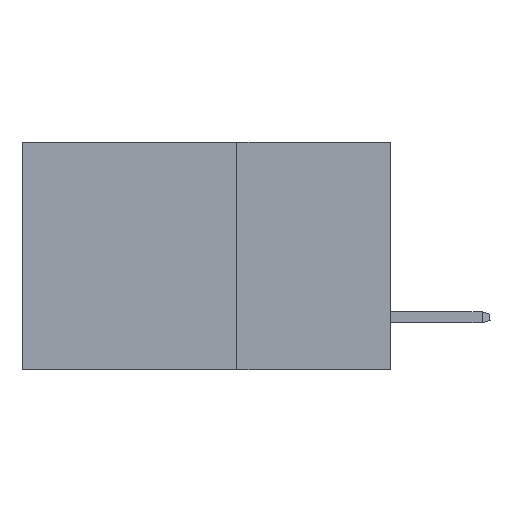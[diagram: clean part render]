
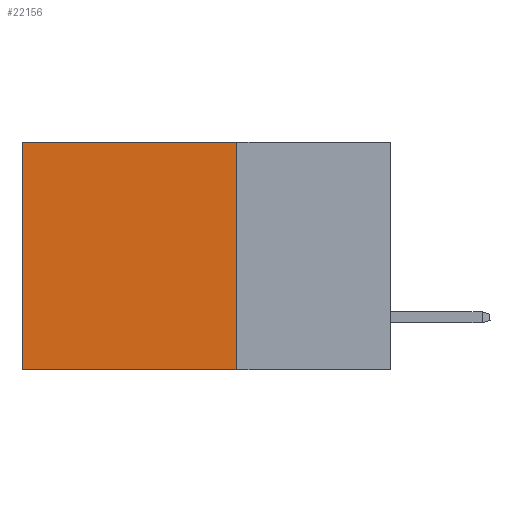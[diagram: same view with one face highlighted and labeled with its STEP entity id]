
A CAD part, left-side view. The second image highlights one B-rep face of the part: STEP entity #22156.
In plain terms, the highlighted planar face has unit normal (-1, 0, 0).
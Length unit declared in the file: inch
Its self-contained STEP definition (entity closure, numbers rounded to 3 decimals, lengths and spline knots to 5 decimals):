
#154 = LINE ( 'NONE', #38061, #28323 ) ;
#233 = CARTESIAN_POINT ( 'NONE',  ( 0.2875, 0.25, 0. ) ) ;
#596 = DIRECTION ( 'NONE',  ( 1., 0., 0. ) ) ;
#2822 = DIRECTION ( 'NONE',  ( 0., 1., 0. ) ) ;
#3446 = AXIS2_PLACEMENT_3D ( 'NONE', #34140, #596, #27820 ) ;
#3474 = ORIENTED_EDGE ( 'NONE', *, *, #25304, .T. ) ;
#4267 = CARTESIAN_POINT ( 'NONE',  ( 0.2875, 0.6, 0. ) ) ;
#4730 = ORIENTED_EDGE ( 'NONE', *, *, #14079, .F. ) ;
#5203 = CARTESIAN_POINT ( 'NONE',  ( 0.2875, 0.6, -0.37 ) ) ;
#5903 = CARTESIAN_POINT ( 'NONE',  ( 0.2875, 0.25, 0. ) ) ;
#7310 = DIRECTION ( 'NONE',  ( 0., 0., -1. ) ) ;
#7563 = LINE ( 'NONE', #25969, #22406 ) ;
#9550 = EDGE_CURVE ( 'NONE', #39349, #24073, #13376, .T. ) ;
#11528 = FACE_OUTER_BOUND ( 'NONE', #12274, .T. ) ;
#12274 = EDGE_LOOP ( 'NONE', ( #20161, #17714, #4730, #3474 ) ) ;
#12705 = CARTESIAN_POINT ( 'NONE',  ( 0.2875, 0.6, 0. ) ) ;
#13376 = LINE ( 'NONE', #4267, #39272 ) ;
#14079 = EDGE_CURVE ( 'NONE', #20731, #23563, #7563, .T. ) ;
#16460 = VECTOR ( 'NONE', #2822, 39.37008 ) ;
#17714 = ORIENTED_EDGE ( 'NONE', *, *, #30950, .F. ) ;
#20161 = ORIENTED_EDGE ( 'NONE', *, *, #9550, .T. ) ;
#20731 = VERTEX_POINT ( 'NONE', #233 ) ;
#22156 = ADVANCED_FACE ( 'NONE', ( #11528 ), #37015, .F. ) ;
#22406 = VECTOR ( 'NONE', #34810, 39.37008 ) ;
#23563 = VERTEX_POINT ( 'NONE', #27569 ) ;
#24073 = VERTEX_POINT ( 'NONE', #5203 ) ;
#25304 = EDGE_CURVE ( 'NONE', #20731, #39349, #25990, .T. ) ;
#25969 = CARTESIAN_POINT ( 'NONE',  ( 0.2875, 0.25, 0. ) ) ;
#25990 = LINE ( 'NONE', #5903, #16460 ) ;
#27569 = CARTESIAN_POINT ( 'NONE',  ( 0.2875, 0.25, -0.37 ) ) ;
#27820 = DIRECTION ( 'NONE',  ( 0., 0., -1. ) ) ;
#28323 = VECTOR ( 'NONE', #28740, 39.37008 ) ;
#28740 = DIRECTION ( 'NONE',  ( 0., 1., 0. ) ) ;
#30950 = EDGE_CURVE ( 'NONE', #23563, #24073, #154, .T. ) ;
#34140 = CARTESIAN_POINT ( 'NONE',  ( 0.2875, 0.25, 0. ) ) ;
#34810 = DIRECTION ( 'NONE',  ( 0., 0., -1. ) ) ;
#37015 = PLANE ( 'NONE',  #3446 ) ;
#38061 = CARTESIAN_POINT ( 'NONE',  ( 0.2875, 0.25, -0.37 ) ) ;
#39272 = VECTOR ( 'NONE', #7310, 39.37008 ) ;
#39349 = VERTEX_POINT ( 'NONE', #12705 ) ;
